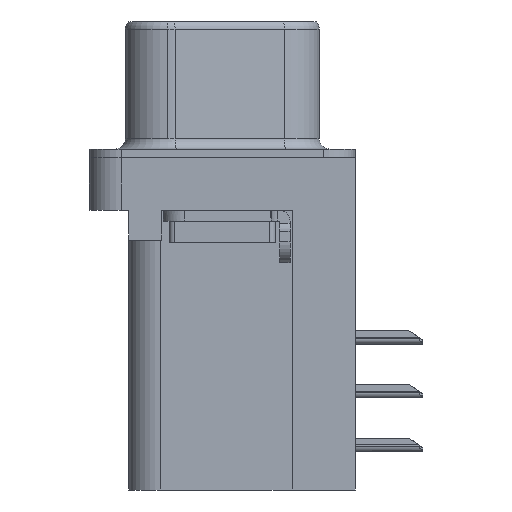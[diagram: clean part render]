
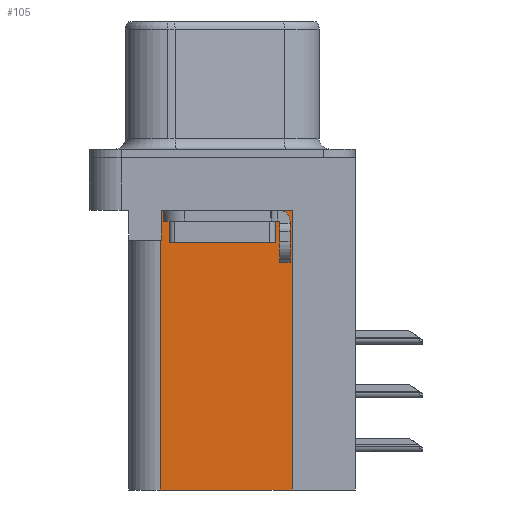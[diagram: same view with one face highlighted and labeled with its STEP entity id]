
A CAD part, left-side view. The second image highlights one B-rep face of the part: STEP entity #105.
In plain terms, the highlighted planar face has unit normal (-1, 0, 0).
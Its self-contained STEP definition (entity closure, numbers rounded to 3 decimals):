
#41 = CARTESIAN_POINT ( 'NONE',  ( 3.7, 2.895, -3.9 ) ) ;
#78 = EDGE_CURVE ( 'NONE', #22374, #12583, #28704, .T. ) ;
#105 = ADVANCED_FACE ( 'NONE', ( #10103 ), #5886, .F. ) ;
#258 = DIRECTION ( 'NONE',  ( 0., 1., 0. ) ) ;
#387 = VECTOR ( 'NONE', #2302, 1000. ) ;
#2302 = DIRECTION ( 'NONE',  ( 0., 0., 1. ) ) ;
#3186 = CARTESIAN_POINT ( 'NONE',  ( 3.7, 2.925, -15.7 ) ) ;
#4013 = VECTOR ( 'NONE', #7673, 1000. ) ;
#4095 = AXIS2_PLACEMENT_3D ( 'NONE', #5880, #5948, #5987 ) ;
#4229 = DIRECTION ( 'NONE',  ( 0., 1., 0. ) ) ;
#4804 = EDGE_LOOP ( 'NONE', ( #13520, #5442, #20406, #14048, #13065, #25504 ) ) ;
#4876 = VERTEX_POINT ( 'NONE', #21621 ) ;
#5021 = CARTESIAN_POINT ( 'NONE',  ( 3.7, 2.925, -3.9 ) ) ;
#5442 = ORIENTED_EDGE ( 'NONE', *, *, #9928, .T. ) ;
#5880 = CARTESIAN_POINT ( 'NONE',  ( 3.7, -3.295, -15.7 ) ) ;
#5886 = PLANE ( 'NONE',  #4095 ) ;
#5948 = DIRECTION ( 'NONE',  ( 1., 0., 0. ) ) ;
#5987 = DIRECTION ( 'NONE',  ( 0., 0., -1. ) ) ;
#6014 = LINE ( 'NONE', #17767, #13510 ) ;
#6396 = LINE ( 'NONE', #15846, #387 ) ;
#7072 = CARTESIAN_POINT ( 'NONE',  ( 3.7, -3.295, -2.5 ) ) ;
#7503 = VECTOR ( 'NONE', #258, 1000. ) ;
#7673 = DIRECTION ( 'NONE',  ( 0., 0., 1. ) ) ;
#7838 = CARTESIAN_POINT ( 'NONE',  ( 3.7, 2.925, -15.7 ) ) ;
#9928 = EDGE_CURVE ( 'NONE', #4876, #27651, #14232, .T. ) ;
#10103 = FACE_OUTER_BOUND ( 'NONE', #4804, .T. ) ;
#10516 = EDGE_CURVE ( 'NONE', #22144, #22374, #6014, .T. ) ;
#10961 = LINE ( 'NONE', #15734, #27408 ) ;
#11270 = CARTESIAN_POINT ( 'NONE',  ( 3.7, -3.295, -15.7 ) ) ;
#11911 = EDGE_CURVE ( 'NONE', #27651, #12583, #10961, .T. ) ;
#12583 = VERTEX_POINT ( 'NONE', #5021 ) ;
#13065 = ORIENTED_EDGE ( 'NONE', *, *, #10516, .F. ) ;
#13510 = VECTOR ( 'NONE', #4229, 1000. ) ;
#13520 = ORIENTED_EDGE ( 'NONE', *, *, #16160, .T. ) ;
#13607 = CARTESIAN_POINT ( 'NONE',  ( 3.7, 2.895, -3.9 ) ) ;
#14048 = ORIENTED_EDGE ( 'NONE', *, *, #78, .F. ) ;
#14232 = LINE ( 'NONE', #41, #26114 ) ;
#15734 = CARTESIAN_POINT ( 'NONE',  ( 3.7, 0., -3.9 ) ) ;
#15832 = DIRECTION ( 'NONE',  ( 0., 0., -1. ) ) ;
#15846 = CARTESIAN_POINT ( 'NONE',  ( 3.7, -3.295, -15.7 ) ) ;
#16160 = EDGE_CURVE ( 'NONE', #20593, #4876, #24751, .T. ) ;
#17767 = CARTESIAN_POINT ( 'NONE',  ( 3.7, -3.295, -15.7 ) ) ;
#20406 = ORIENTED_EDGE ( 'NONE', *, *, #11911, .T. ) ;
#20593 = VERTEX_POINT ( 'NONE', #20943 ) ;
#20943 = CARTESIAN_POINT ( 'NONE',  ( 3.7, -3.295, -2.5 ) ) ;
#21621 = CARTESIAN_POINT ( 'NONE',  ( 3.7, 2.895, -2.5 ) ) ;
#22144 = VERTEX_POINT ( 'NONE', #11270 ) ;
#22173 = EDGE_CURVE ( 'NONE', #22144, #20593, #6396, .T. ) ;
#22374 = VERTEX_POINT ( 'NONE', #3186 ) ;
#22482 = DIRECTION ( 'NONE',  ( 0., 1., 0. ) ) ;
#24751 = LINE ( 'NONE', #7072, #7503 ) ;
#25504 = ORIENTED_EDGE ( 'NONE', *, *, #22173, .T. ) ;
#26114 = VECTOR ( 'NONE', #15832, 1000. ) ;
#27408 = VECTOR ( 'NONE', #22482, 1000. ) ;
#27651 = VERTEX_POINT ( 'NONE', #13607 ) ;
#28704 = LINE ( 'NONE', #7838, #4013 ) ;
